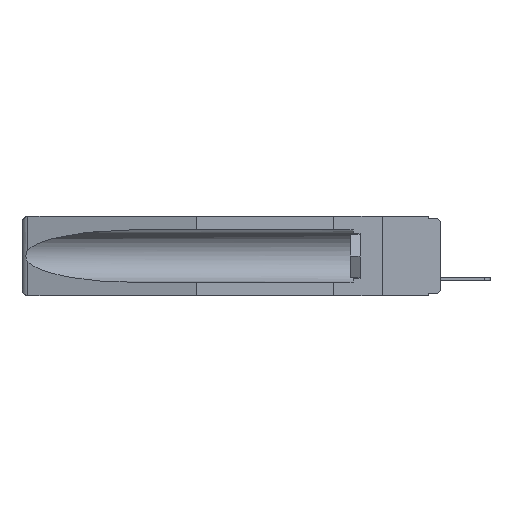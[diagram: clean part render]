
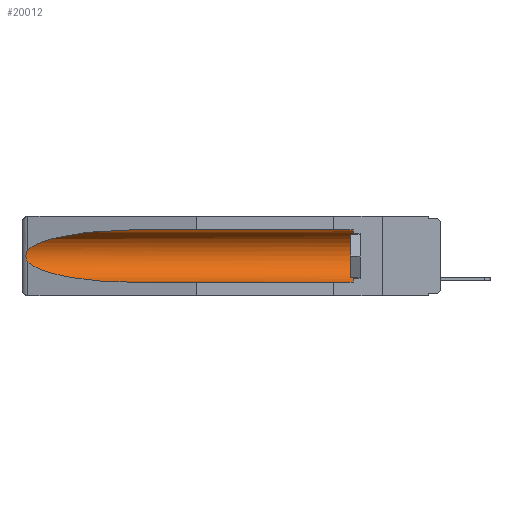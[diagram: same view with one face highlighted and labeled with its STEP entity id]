
A CAD part, left-side view. The second image highlights one B-rep face of the part: STEP entity #20012.
In plain terms, the highlighted cylindrical face has radius 2.857 mm (diameter 5.715 mm), a partial arc.
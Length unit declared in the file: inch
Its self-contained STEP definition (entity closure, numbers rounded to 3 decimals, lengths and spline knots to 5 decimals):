
#55 = B_SPLINE_CURVE_WITH_KNOTS ( 'NONE', 3,
 ( #5981, #12095, #11994, #10464, #8746, #15040, #2855, #7314, #13424, #18114 ),
 .UNSPECIFIED., .F., .F.,
 ( 4, 2, 2, 2, 4 ),
 ( 0., 0.00029, 0.00058, 0.00087, 0.00117 ),
 .UNSPECIFIED. ) ;
#376 = CARTESIAN_POINT ( 'NONE',  ( 0.25451, 1.48313, -0.09465 ) ) ;
#606 = EDGE_CURVE ( 'NONE', #17938, #7173, #55, .T. ) ;
#783 = EDGE_LOOP ( 'NONE', ( #13387, #1094, #5724, #3283, #1582, #1896 ) ) ;
#1094 = ORIENTED_EDGE ( 'NONE', *, *, #606, .T. ) ;
#1137 = CIRCLE ( 'NONE', #18336, 0.1125 ) ;
#1415 = CARTESIAN_POINT ( 'NONE',  ( 0.155, 0.126, -0.1715 ) ) ;
#1552 = FACE_OUTER_BOUND ( 'NONE', #783, .T. ) ;
#1582 = ORIENTED_EDGE ( 'NONE', *, *, #4795, .T. ) ;
#1650 = DIRECTION ( 'NONE',  ( 0., 0., 1. ) ) ;
#1896 = ORIENTED_EDGE ( 'NONE', *, *, #19749, .T. ) ;
#2355 = CARTESIAN_POINT ( 'NONE',  ( 0.21114, 1.30732, -0.284 ) ) ;
#2855 = CARTESIAN_POINT ( 'NONE',  ( 0.2673, 1.53269, -0.17917 ) ) ;
#3283 = ORIENTED_EDGE ( 'NONE', *, *, #17745, .F. ) ;
#3451 = DIRECTION ( 'NONE',  ( 0., 1., 0. ) ) ;
#3667 = LINE ( 'NONE', #19250, #4132 ) ;
#3702 = VERTEX_POINT ( 'NONE', #17157 ) ;
#3880 = CARTESIAN_POINT ( 'NONE',  ( 0.155, 1.07973, -0.284 ) ) ;
#4132 = VECTOR ( 'NONE', #16384, 39.37008 ) ;
#4341 = DIRECTION ( 'NONE',  ( 0., 0., 1. ) ) ;
#4795 = EDGE_CURVE ( 'NONE', #3702, #9189, #1137, .T. ) ;
#4903 = EDGE_CURVE ( 'NONE', #11162, #17938, #15258, .T. ) ;
#5023 = CARTESIAN_POINT ( 'NONE',  ( 0.26537, 1.52718, -0.14972 ) ) ;
#5724 = ORIENTED_EDGE ( 'NONE', *, *, #19720, .T. ) ;
#5901 = CARTESIAN_POINT ( 'NONE',  ( 0.26537, 1.52718, -0.19328 ) ) ;
#5981 = CARTESIAN_POINT ( 'NONE',  ( 0.26537, 1.52718, -0.14972 ) ) ;
#6081 = AXIS2_PLACEMENT_3D ( 'NONE', #8024, #3451, #1650 ) ;
#6261 = VERTEX_POINT ( 'NONE', #14836 ) ;
#6277 =( BOUNDED_CURVE ( )  B_SPLINE_CURVE ( 3, ( #14442, #17821, #2355, #3880 ),
 .UNSPECIFIED., .F., .F. ) 
 B_SPLINE_CURVE_WITH_KNOTS ( ( 4, 4 ),
 ( 0.1948, 1.5708 ),
 .UNSPECIFIED. ) 
 CURVE ( )  GEOMETRIC_REPRESENTATION_ITEM ( )  RATIONAL_B_SPLINE_CURVE ( ( 1., 0.848, 0.848, 1. ) ) 
 REPRESENTATION_ITEM ( '' )  );
#6506 = CARTESIAN_POINT ( 'NONE',  ( 0.155, 1.07973, -0.059 ) ) ;
#7173 = VERTEX_POINT ( 'NONE', #5901 ) ;
#7314 = CARTESIAN_POINT ( 'NONE',  ( 0.26655, 1.53094, -0.18657 ) ) ;
#8024 = CARTESIAN_POINT ( 'NONE',  ( 0.155, -0.30754, -0.1715 ) ) ;
#8746 = CARTESIAN_POINT ( 'NONE',  ( 0.2675, 1.53308, -0.16763 ) ) ;
#9189 = VERTEX_POINT ( 'NONE', #11555 ) ;
#9554 = CYLINDRICAL_SURFACE ( 'NONE', #6081, 0.1125 ) ;
#10464 = CARTESIAN_POINT ( 'NONE',  ( 0.2673, 1.5327, -0.16383 ) ) ;
#11162 = VERTEX_POINT ( 'NONE', #6506 ) ;
#11555 = CARTESIAN_POINT ( 'NONE',  ( 0.155, 0.126, -0.059 ) ) ;
#11994 = CARTESIAN_POINT ( 'NONE',  ( 0.26654, 1.53092, -0.15636 ) ) ;
#12095 = CARTESIAN_POINT ( 'NONE',  ( 0.26597, 1.52961, -0.15275 ) ) ;
#13387 = ORIENTED_EDGE ( 'NONE', *, *, #4903, .T. ) ;
#13424 = CARTESIAN_POINT ( 'NONE',  ( 0.26597, 1.5296, -0.19026 ) ) ;
#13788 = CARTESIAN_POINT ( 'NONE',  ( 0.155, -0.30754, -0.284 ) ) ;
#13821 = VECTOR ( 'NONE', #20000, 39.37008 ) ;
#14442 = CARTESIAN_POINT ( 'NONE',  ( 0.26537, 1.52718, -0.19328 ) ) ;
#14836 = CARTESIAN_POINT ( 'NONE',  ( 0.155, 1.07973, -0.284 ) ) ;
#15040 = CARTESIAN_POINT ( 'NONE',  ( 0.2675, 1.53308, -0.17534 ) ) ;
#15258 =( BOUNDED_CURVE ( )  B_SPLINE_CURVE ( 3, ( #20016, #15813, #376, #5023 ),
 .UNSPECIFIED., .F., .F. ) 
 B_SPLINE_CURVE_WITH_KNOTS ( ( 4, 4 ),
 ( 4.71239, 6.08839 ),
 .UNSPECIFIED. ) 
 CURVE ( )  GEOMETRIC_REPRESENTATION_ITEM ( )  RATIONAL_B_SPLINE_CURVE ( ( 1., 0.848, 0.848, 1. ) ) 
 REPRESENTATION_ITEM ( '' )  );
#15813 = CARTESIAN_POINT ( 'NONE',  ( 0.21114, 1.30732, -0.059 ) ) ;
#16384 = DIRECTION ( 'NONE',  ( 0., 1., 0. ) ) ;
#17157 = CARTESIAN_POINT ( 'NONE',  ( 0.155, 0.126, -0.284 ) ) ;
#17745 = EDGE_CURVE ( 'NONE', #3702, #6261, #19904, .T. ) ;
#17821 = CARTESIAN_POINT ( 'NONE',  ( 0.25451, 1.48313, -0.24835 ) ) ;
#17938 = VERTEX_POINT ( 'NONE', #18666 ) ;
#18114 = CARTESIAN_POINT ( 'NONE',  ( 0.26537, 1.52718, -0.19328 ) ) ;
#18286 = DIRECTION ( 'NONE',  ( 0., -1., 0. ) ) ;
#18336 = AXIS2_PLACEMENT_3D ( 'NONE', #1415, #18286, #4341 ) ;
#18666 = CARTESIAN_POINT ( 'NONE',  ( 0.26537, 1.52718, -0.14972 ) ) ;
#19250 = CARTESIAN_POINT ( 'NONE',  ( 0.155, -0.30754, -0.059 ) ) ;
#19720 = EDGE_CURVE ( 'NONE', #7173, #6261, #6277, .T. ) ;
#19749 = EDGE_CURVE ( 'NONE', #9189, #11162, #3667, .T. ) ;
#19904 = LINE ( 'NONE', #13788, #13821 ) ;
#20000 = DIRECTION ( 'NONE',  ( 0., 1., 0. ) ) ;
#20012 = ADVANCED_FACE ( 'NONE', ( #1552 ), #9554, .F. ) ;
#20016 = CARTESIAN_POINT ( 'NONE',  ( 0.155, 1.07973, -0.059 ) ) ;
